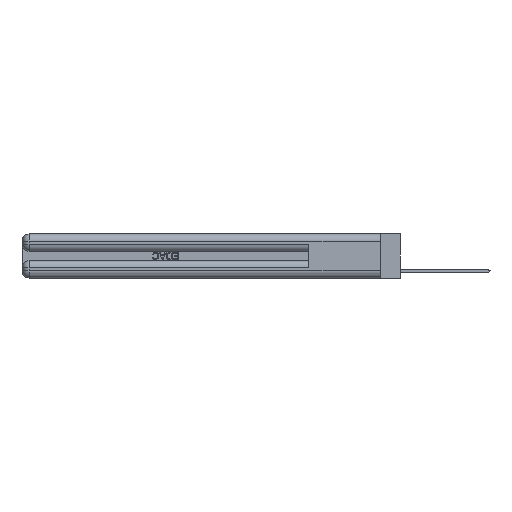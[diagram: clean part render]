
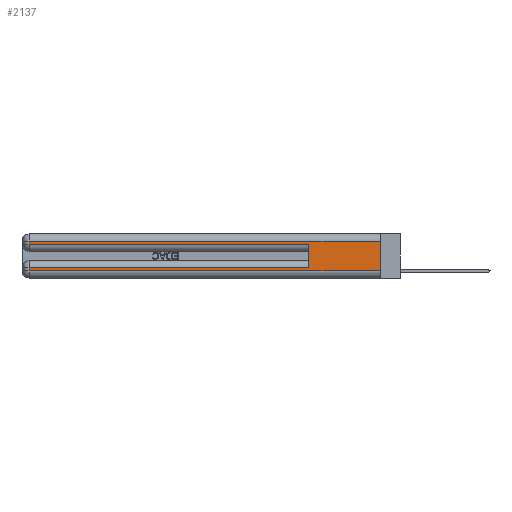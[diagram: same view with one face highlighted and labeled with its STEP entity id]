
A CAD part, left-side view. The second image highlights one B-rep face of the part: STEP entity #2137.
In plain terms, the highlighted planar face has unit normal (-1, 0, 0).
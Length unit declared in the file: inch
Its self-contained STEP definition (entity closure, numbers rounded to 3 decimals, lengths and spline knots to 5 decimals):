
#766 = DIRECTION ( 'NONE',  ( 0., -1., 0. ) ) ;
#1057 = LINE ( 'NONE', #9603, #13061 ) ;
#2137 = ADVANCED_FACE ( 'NONE', ( #22410 ), #33271, .F. ) ;
#2812 = ORIENTED_EDGE ( 'NONE', *, *, #20067, .F. ) ;
#2997 = CARTESIAN_POINT ( 'NONE',  ( 0., 2.94, 0.31 ) ) ;
#3005 = CARTESIAN_POINT ( 'NONE',  ( 0., 0.6, 0.145 ) ) ;
#3423 = CARTESIAN_POINT ( 'NONE',  ( 0., 0., 0.06 ) ) ;
#3540 = CARTESIAN_POINT ( 'NONE',  ( 0., 0., 0.31 ) ) ;
#3669 = CARTESIAN_POINT ( 'NONE',  ( 0., 0., 0.37 ) ) ;
#4147 = VECTOR ( 'NONE', #766, 39.37008 ) ;
#4401 = DIRECTION ( 'NONE',  ( 0., 0., -1. ) ) ;
#5461 = DIRECTION ( 'NONE',  ( 0., 0., -1. ) ) ;
#5515 = EDGE_CURVE ( 'NONE', #19102, #21605, #10684, .T. ) ;
#5793 = VERTEX_POINT ( 'NONE', #25482 ) ;
#6166 = DIRECTION ( 'NONE',  ( 1., 0., 0. ) ) ;
#6903 = LINE ( 'NONE', #17816, #12041 ) ;
#8195 = DIRECTION ( 'NONE',  ( 0., -1., 0. ) ) ;
#9443 = VERTEX_POINT ( 'NONE', #28816 ) ;
#9603 = CARTESIAN_POINT ( 'NONE',  ( 0., 0., 0.085 ) ) ;
#10249 = ORIENTED_EDGE ( 'NONE', *, *, #26796, .T. ) ;
#10684 = LINE ( 'NONE', #3540, #32308 ) ;
#10858 = VERTEX_POINT ( 'NONE', #16520 ) ;
#10873 = EDGE_CURVE ( 'NONE', #27759, #10858, #33265, .T. ) ;
#11197 = VERTEX_POINT ( 'NONE', #19510 ) ;
#12041 = VECTOR ( 'NONE', #4401, 39.37008 ) ;
#12100 = EDGE_CURVE ( 'NONE', #9443, #5793, #27429, .T. ) ;
#12138 = CARTESIAN_POINT ( 'NONE',  ( 0., 2.94, 0.085 ) ) ;
#12910 = ORIENTED_EDGE ( 'NONE', *, *, #17104, .T. ) ;
#13061 = VECTOR ( 'NONE', #30820, 39.37008 ) ;
#16250 = ORIENTED_EDGE ( 'NONE', *, *, #17026, .T. ) ;
#16470 = VECTOR ( 'NONE', #8195, 39.37008 ) ;
#16520 = CARTESIAN_POINT ( 'NONE',  ( 0., 2.94, 0.06 ) ) ;
#16839 = EDGE_LOOP ( 'NONE', ( #2812, #23231, #10249, #16250, #30348, #12910, #19383, #33994 ) ) ;
#17026 = EDGE_CURVE ( 'NONE', #11197, #5793, #32625, .T. ) ;
#17068 = DIRECTION ( 'NONE',  ( 0., 0., -1. ) ) ;
#17104 = EDGE_CURVE ( 'NONE', #9443, #27759, #1057, .T. ) ;
#17816 = CARTESIAN_POINT ( 'NONE',  ( 0., 0., 0.37 ) ) ;
#19102 = VERTEX_POINT ( 'NONE', #31843 ) ;
#19383 = ORIENTED_EDGE ( 'NONE', *, *, #10873, .T. ) ;
#19510 = CARTESIAN_POINT ( 'NONE',  ( 0., 2.94, 0.285 ) ) ;
#20067 = EDGE_CURVE ( 'NONE', #19102, #23286, #6903, .T. ) ;
#20434 = CARTESIAN_POINT ( 'NONE',  ( 0., 2.94, 0.37 ) ) ;
#21359 = EDGE_CURVE ( 'NONE', #10858, #23286, #30523, .T. ) ;
#21605 = VERTEX_POINT ( 'NONE', #2997 ) ;
#22410 = FACE_OUTER_BOUND ( 'NONE', #16839, .T. ) ;
#23231 = ORIENTED_EDGE ( 'NONE', *, *, #5515, .T. ) ;
#23286 = VERTEX_POINT ( 'NONE', #26564 ) ;
#24772 = DIRECTION ( 'NONE',  ( 0., 1., 0. ) ) ;
#24933 = DIRECTION ( 'NONE',  ( 0., 0., 1. ) ) ;
#25482 = CARTESIAN_POINT ( 'NONE',  ( 0., 0.6, 0.285 ) ) ;
#26564 = CARTESIAN_POINT ( 'NONE',  ( 0., 0., 0.06 ) ) ;
#26796 = EDGE_CURVE ( 'NONE', #21605, #11197, #32557, .T. ) ;
#27271 = CARTESIAN_POINT ( 'NONE',  ( 0., 0., 0.285 ) ) ;
#27429 = LINE ( 'NONE', #3005, #33819 ) ;
#27453 = VECTOR ( 'NONE', #34144, 39.37008 ) ;
#27759 = VERTEX_POINT ( 'NONE', #12138 ) ;
#28816 = CARTESIAN_POINT ( 'NONE',  ( 0., 0.6, 0.085 ) ) ;
#30348 = ORIENTED_EDGE ( 'NONE', *, *, #12100, .F. ) ;
#30523 = LINE ( 'NONE', #3423, #4147 ) ;
#30820 = DIRECTION ( 'NONE',  ( 0., 1., 0. ) ) ;
#30849 = AXIS2_PLACEMENT_3D ( 'NONE', #3669, #6166, #17068 ) ;
#31695 = VECTOR ( 'NONE', #5461, 39.37008 ) ;
#31843 = CARTESIAN_POINT ( 'NONE',  ( 0., 0., 0.31 ) ) ;
#32308 = VECTOR ( 'NONE', #24772, 39.37008 ) ;
#32557 = LINE ( 'NONE', #34457, #31695 ) ;
#32625 = LINE ( 'NONE', #27271, #16470 ) ;
#33265 = LINE ( 'NONE', #20434, #27453 ) ;
#33271 = PLANE ( 'NONE',  #30849 ) ;
#33819 = VECTOR ( 'NONE', #24933, 39.37008 ) ;
#33994 = ORIENTED_EDGE ( 'NONE', *, *, #21359, .T. ) ;
#34144 = DIRECTION ( 'NONE',  ( 0., 0., -1. ) ) ;
#34457 = CARTESIAN_POINT ( 'NONE',  ( 0., 2.94, 0.37 ) ) ;
